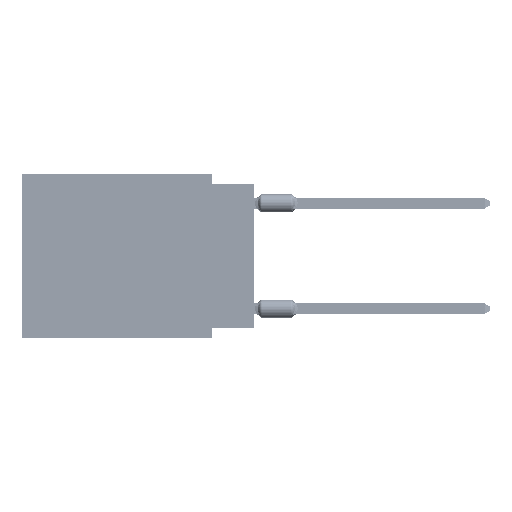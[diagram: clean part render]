
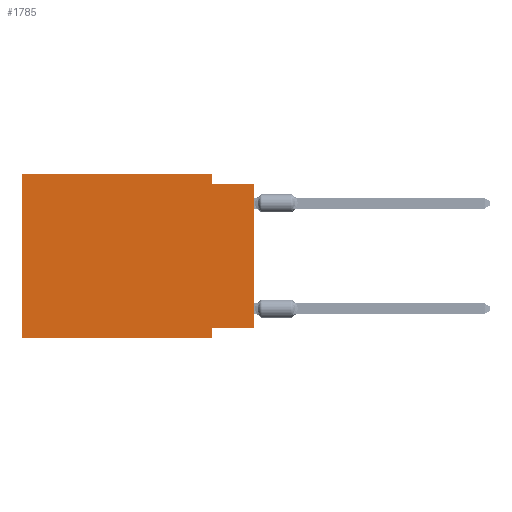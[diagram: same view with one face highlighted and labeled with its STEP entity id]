
A CAD part, left-side view. The second image highlights one B-rep face of the part: STEP entity #1785.
In plain terms, the highlighted planar face has unit normal (-1, 0, 0).
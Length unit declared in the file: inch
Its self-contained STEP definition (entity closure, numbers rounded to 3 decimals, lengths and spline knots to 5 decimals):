
#416 = DIRECTION ( 'NONE',  ( 0., 0., -1. ) ) ;
#1517 = ORIENTED_EDGE ( 'NONE', *, *, #38067, .F. ) ;
#1785 = ADVANCED_FACE ( 'NONE', ( #55855 ), #40496, .F. ) ;
#2293 = ORIENTED_EDGE ( 'NONE', *, *, #41456, .F. ) ;
#3421 = VERTEX_POINT ( 'NONE', #18668 ) ;
#4373 = LINE ( 'NONE', #58563, #37973 ) ;
#4834 = VERTEX_POINT ( 'NONE', #25402 ) ;
#5029 = DIRECTION ( 'NONE',  ( 0., -1., 0. ) ) ;
#6893 = LINE ( 'NONE', #28622, #53203 ) ;
#7018 = DIRECTION ( 'NONE',  ( 0., 0., -1. ) ) ;
#7217 = CARTESIAN_POINT ( 'NONE',  ( 0., 0.55, -0.39 ) ) ;
#7377 = AXIS2_PLACEMENT_3D ( 'NONE', #34460, #50859, #7018 ) ;
#8578 = VERTEX_POINT ( 'NONE', #46848 ) ;
#8964 = ORIENTED_EDGE ( 'NONE', *, *, #17458, .F. ) ;
#10248 = VERTEX_POINT ( 'NONE', #36063 ) ;
#10769 = VECTOR ( 'NONE', #47620, 39.37008 ) ;
#12203 = VERTEX_POINT ( 'NONE', #7217 ) ;
#12228 = DIRECTION ( 'NONE',  ( 0., 0., 1. ) ) ;
#12969 = VERTEX_POINT ( 'NONE', #28448 ) ;
#14691 = VECTOR ( 'NONE', #42729, 39.37008 ) ;
#14709 = DIRECTION ( 'NONE',  ( 0., 0., 1. ) ) ;
#17458 = EDGE_CURVE ( 'NONE', #3421, #12969, #47379, .T. ) ;
#17636 = VECTOR ( 'NONE', #25179, 39.37008 ) ;
#18668 = CARTESIAN_POINT ( 'NONE',  ( 0., 0.1, 0. ) ) ;
#20849 = LINE ( 'NONE', #35499, #10769 ) ;
#21065 = VECTOR ( 'NONE', #59857, 39.37008 ) ;
#22691 = VERTEX_POINT ( 'NONE', #41115 ) ;
#23727 = ORIENTED_EDGE ( 'NONE', *, *, #56456, .F. ) ;
#25179 = DIRECTION ( 'NONE',  ( 0., -1., 0. ) ) ;
#25392 = LINE ( 'NONE', #47162, #46053 ) ;
#25398 = EDGE_CURVE ( 'NONE', #4834, #10248, #6893, .T. ) ;
#25402 = CARTESIAN_POINT ( 'NONE',  ( 0., 0., -0.365 ) ) ;
#28448 = CARTESIAN_POINT ( 'NONE',  ( 0., 0.1, -0.025 ) ) ;
#28622 = CARTESIAN_POINT ( 'NONE',  ( 0., 0., 0. ) ) ;
#32122 = CARTESIAN_POINT ( 'NONE',  ( 0., 0.55, -0.39 ) ) ;
#34460 = CARTESIAN_POINT ( 'NONE',  ( 0., 0.55, 0. ) ) ;
#35499 = CARTESIAN_POINT ( 'NONE',  ( 0., 0., -0.365 ) ) ;
#36063 = CARTESIAN_POINT ( 'NONE',  ( 0., 0., -0.025 ) ) ;
#37973 = VECTOR ( 'NONE', #416, 39.37008 ) ;
#38067 = EDGE_CURVE ( 'NONE', #8578, #22691, #4373, .T. ) ;
#39307 = EDGE_CURVE ( 'NONE', #12203, #65836, #25392, .T. ) ;
#40496 = PLANE ( 'NONE',  #7377 ) ;
#41115 = CARTESIAN_POINT ( 'NONE',  ( 0., 0.1, -0.39 ) ) ;
#41456 = EDGE_CURVE ( 'NONE', #65836, #3421, #44507, .T. ) ;
#42025 = CARTESIAN_POINT ( 'NONE',  ( 0., 0.55, 0. ) ) ;
#42729 = DIRECTION ( 'NONE',  ( 0., 0., -1. ) ) ;
#44507 = LINE ( 'NONE', #65196, #21065 ) ;
#46053 = VECTOR ( 'NONE', #14709, 39.37008 ) ;
#46848 = CARTESIAN_POINT ( 'NONE',  ( 0., 0.1, -0.365 ) ) ;
#47162 = CARTESIAN_POINT ( 'NONE',  ( 0., 0.55, 0. ) ) ;
#47379 = LINE ( 'NONE', #69104, #14691 ) ;
#47620 = DIRECTION ( 'NONE',  ( 0., 1., 0. ) ) ;
#49069 = EDGE_LOOP ( 'NONE', ( #52932, #61465, #8964, #2293, #67279, #60817, #1517, #23727 ) ) ;
#49491 = VECTOR ( 'NONE', #5029, 39.37008 ) ;
#50859 = DIRECTION ( 'NONE',  ( 1., 0., 0. ) ) ;
#52623 = CARTESIAN_POINT ( 'NONE',  ( 0., 0., -0.025 ) ) ;
#52932 = ORIENTED_EDGE ( 'NONE', *, *, #25398, .T. ) ;
#53203 = VECTOR ( 'NONE', #12228, 39.37008 ) ;
#54099 = EDGE_CURVE ( 'NONE', #12203, #22691, #55249, .T. ) ;
#54805 = EDGE_CURVE ( 'NONE', #12969, #10248, #58005, .T. ) ;
#55249 = LINE ( 'NONE', #32122, #49491 ) ;
#55855 = FACE_OUTER_BOUND ( 'NONE', #49069, .T. ) ;
#56456 = EDGE_CURVE ( 'NONE', #4834, #8578, #20849, .T. ) ;
#58005 = LINE ( 'NONE', #52623, #17636 ) ;
#58563 = CARTESIAN_POINT ( 'NONE',  ( 0., 0.1, -0.39 ) ) ;
#59857 = DIRECTION ( 'NONE',  ( 0., -1., 0. ) ) ;
#60817 = ORIENTED_EDGE ( 'NONE', *, *, #54099, .T. ) ;
#61465 = ORIENTED_EDGE ( 'NONE', *, *, #54805, .F. ) ;
#65196 = CARTESIAN_POINT ( 'NONE',  ( 0., 0.55, 0. ) ) ;
#65836 = VERTEX_POINT ( 'NONE', #42025 ) ;
#67279 = ORIENTED_EDGE ( 'NONE', *, *, #39307, .F. ) ;
#69104 = CARTESIAN_POINT ( 'NONE',  ( 0., 0.1, 0. ) ) ;
